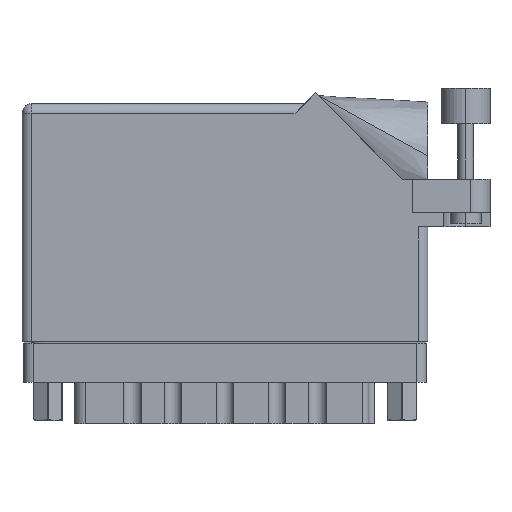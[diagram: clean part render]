
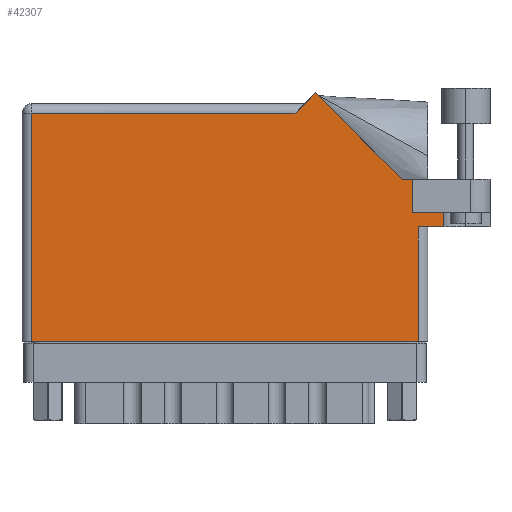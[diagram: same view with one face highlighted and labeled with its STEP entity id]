
A CAD part, front view. The second image highlights one B-rep face of the part: STEP entity #42307.
In plain terms, the highlighted face is planar.
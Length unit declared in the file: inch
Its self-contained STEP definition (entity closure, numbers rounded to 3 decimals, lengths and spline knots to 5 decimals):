
#83 = CARTESIAN_POINT ( 'NONE',  ( 2.7135, 0.737, 0. ) ) ;
#1959 = LINE ( 'NONE', #8560, #41216 ) ;
#4508 = ORIENTED_EDGE ( 'NONE', *, *, #19760, .T. ) ;
#6870 = CARTESIAN_POINT ( 'NONE',  ( 0.062, 1.468, 0. ) ) ;
#8151 = DIRECTION ( 'NONE',  ( -1., 0., 0. ) ) ;
#8560 = CARTESIAN_POINT ( 'NONE',  ( 0., 1.468, 0. ) ) ;
#8792 = DIRECTION ( 'NONE',  ( 1., 0., 0. ) ) ;
#8874 = EDGE_CURVE ( 'NONE', #54669, #28642, #57107, .T. ) ;
#9162 = DIRECTION ( 'NONE',  ( 0., -1., 0. ) ) ;
#10837 = VERTEX_POINT ( 'NONE', #83 ) ;
#11204 = VERTEX_POINT ( 'NONE', #30159 ) ;
#12941 = ORIENTED_EDGE ( 'NONE', *, *, #15660, .T. ) ;
#13410 = CARTESIAN_POINT ( 'NONE',  ( 0., 0., 0. ) ) ;
#13802 = CARTESIAN_POINT ( 'NONE',  ( 2.55, 0.737, 0. ) ) ;
#14585 = CARTESIAN_POINT ( 'NONE',  ( 2.612, 0.737, 0. ) ) ;
#15003 = DIRECTION ( 'NONE',  ( 0., -1., 0. ) ) ;
#15450 = DIRECTION ( 'NONE',  ( -1., 0., 0. ) ) ;
#15589 = ORIENTED_EDGE ( 'NONE', *, *, #17703, .T. ) ;
#15660 = EDGE_CURVE ( 'NONE', #30916, #28699, #36635, .T. ) ;
#15791 = LINE ( 'NONE', #17944, #39968 ) ;
#15949 = VECTOR ( 'NONE', #27291, 39.37008 ) ;
#16509 = CARTESIAN_POINT ( 'NONE',  ( 2.512, 0.831, 0. ) ) ;
#17283 = CARTESIAN_POINT ( 'NONE',  ( 1.819, 1.53, 0. ) ) ;
#17703 = EDGE_CURVE ( 'NONE', #53896, #54669, #53895, .T. ) ;
#17736 = CARTESIAN_POINT ( 'NONE',  ( 3.012, 1.044, 0. ) ) ;
#17944 = CARTESIAN_POINT ( 'NONE',  ( 2.44642, 1.044, 0. ) ) ;
#18323 = VECTOR ( 'NONE', #15003, 39.37008 ) ;
#19233 = VERTEX_POINT ( 'NONE', #13802 ) ;
#19760 = EDGE_CURVE ( 'NONE', #28699, #34878, #15791, .T. ) ;
#19881 = CARTESIAN_POINT ( 'NONE',  ( 2.55, 0.737, 0. ) ) ;
#20090 = DIRECTION ( 'NONE',  ( 0., 0., -1. ) ) ;
#20126 = VECTOR ( 'NONE', #26714, 39.37008 ) ;
#21041 = CARTESIAN_POINT ( 'NONE',  ( 0.062, 0., 0. ) ) ;
#21654 = ORIENTED_EDGE ( 'NONE', *, *, #55312, .T. ) ;
#23703 = DIRECTION ( 'NONE',  ( 1., 0., 0. ) ) ;
#26714 = DIRECTION ( 'NONE',  ( 0., 1., 0. ) ) ;
#27186 = VERTEX_POINT ( 'NONE', #39521 ) ;
#27291 = DIRECTION ( 'NONE',  ( -0.707, -0.707, 0. ) ) ;
#27319 = LINE ( 'NONE', #27887, #52255 ) ;
#27728 = DIRECTION ( 'NONE',  ( -1., 0., 0. ) ) ;
#27887 = CARTESIAN_POINT ( 'NONE',  ( 2.512, 0.831, 0. ) ) ;
#28537 = ORIENTED_EDGE ( 'NONE', *, *, #34823, .T. ) ;
#28642 = VERTEX_POINT ( 'NONE', #55098 ) ;
#28699 = VERTEX_POINT ( 'NONE', #41520 ) ;
#28849 = LINE ( 'NONE', #17283, #15949 ) ;
#29623 = PLANE ( 'NONE',  #55949 ) ;
#29969 = EDGE_CURVE ( 'NONE', #34889, #11204, #27319, .T. ) ;
#30159 = CARTESIAN_POINT ( 'NONE',  ( 2.7135, 0.831, 0. ) ) ;
#30261 = ORIENTED_EDGE ( 'NONE', *, *, #57741, .T. ) ;
#30916 = VERTEX_POINT ( 'NONE', #35532 ) ;
#32987 = LINE ( 'NONE', #16509, #20126 ) ;
#33239 = VECTOR ( 'NONE', #54570, 39.37008 ) ;
#33975 = VECTOR ( 'NONE', #9162, 39.37008 ) ;
#34823 = EDGE_CURVE ( 'NONE', #19233, #10837, #61663, .T. ) ;
#34837 = ORIENTED_EDGE ( 'NONE', *, *, #36768, .T. ) ;
#34878 = VERTEX_POINT ( 'NONE', #39264 ) ;
#34889 = VERTEX_POINT ( 'NONE', #38860 ) ;
#35532 = CARTESIAN_POINT ( 'NONE',  ( 2.512, 1.044, 0. ) ) ;
#36635 = LINE ( 'NONE', #17736, #47208 ) ;
#36768 = EDGE_CURVE ( 'NONE', #34878, #27186, #28849, .T. ) ;
#37595 = DIRECTION ( 'NONE',  ( -0.707, 0.707, 0. ) ) ;
#38031 = FACE_OUTER_BOUND ( 'NONE', #61234, .T. ) ;
#38267 = CARTESIAN_POINT ( 'NONE',  ( 2.7135, 1.16177, 0. ) ) ;
#38626 = ORIENTED_EDGE ( 'NONE', *, *, #55184, .F. ) ;
#38860 = CARTESIAN_POINT ( 'NONE',  ( 2.512, 0.831, 0. ) ) ;
#39264 = CARTESIAN_POINT ( 'NONE',  ( 1.88971, 1.60071, 0. ) ) ;
#39521 = CARTESIAN_POINT ( 'NONE',  ( 1.757, 1.468, 0. ) ) ;
#39735 = CARTESIAN_POINT ( 'NONE',  ( 0., 1.53, 0. ) ) ;
#39968 = VECTOR ( 'NONE', #37595, 39.37008 ) ;
#40309 = EDGE_CURVE ( 'NONE', #27186, #53896, #1959, .T. ) ;
#41216 = VECTOR ( 'NONE', #8151, 39.37008 ) ;
#41520 = CARTESIAN_POINT ( 'NONE',  ( 2.44642, 1.044, 0. ) ) ;
#42307 = ADVANCED_FACE ( 'NONE', ( #38031 ), #29623, .F. ) ;
#42448 = ORIENTED_EDGE ( 'NONE', *, *, #29969, .F. ) ;
#44222 = VECTOR ( 'NONE', #23703, 39.37008 ) ;
#47208 = VECTOR ( 'NONE', #27728, 39.37008 ) ;
#52255 = VECTOR ( 'NONE', #61719, 39.37008 ) ;
#53895 = LINE ( 'NONE', #59210, #18323 ) ;
#53896 = VERTEX_POINT ( 'NONE', #6870 ) ;
#54570 = DIRECTION ( 'NONE',  ( 0., 1., 0. ) ) ;
#54669 = VERTEX_POINT ( 'NONE', #21041 ) ;
#55098 = CARTESIAN_POINT ( 'NONE',  ( 2.55, 0., 0. ) ) ;
#55184 = EDGE_CURVE ( 'NONE', #11204, #10837, #60520, .T. ) ;
#55312 = EDGE_CURVE ( 'NONE', #28642, #19233, #55990, .T. ) ;
#55949 = AXIS2_PLACEMENT_3D ( 'NONE', #39735, #20090, #15450 ) ;
#55990 = LINE ( 'NONE', #19881, #33239 ) ;
#57107 = LINE ( 'NONE', #13410, #62386 ) ;
#57741 = EDGE_CURVE ( 'NONE', #34889, #30916, #32987, .T. ) ;
#57943 = ORIENTED_EDGE ( 'NONE', *, *, #40309, .T. ) ;
#59210 = CARTESIAN_POINT ( 'NONE',  ( 0.062, 0., 0. ) ) ;
#59276 = ORIENTED_EDGE ( 'NONE', *, *, #8874, .T. ) ;
#60520 = LINE ( 'NONE', #38267, #33975 ) ;
#61234 = EDGE_LOOP ( 'NONE', ( #59276, #21654, #28537, #38626, #42448, #30261, #12941, #4508, #34837, #57943, #15589 ) ) ;
#61663 = LINE ( 'NONE', #14585, #44222 ) ;
#61719 = DIRECTION ( 'NONE',  ( 1., 0., 0. ) ) ;
#62386 = VECTOR ( 'NONE', #8792, 39.37008 ) ;
